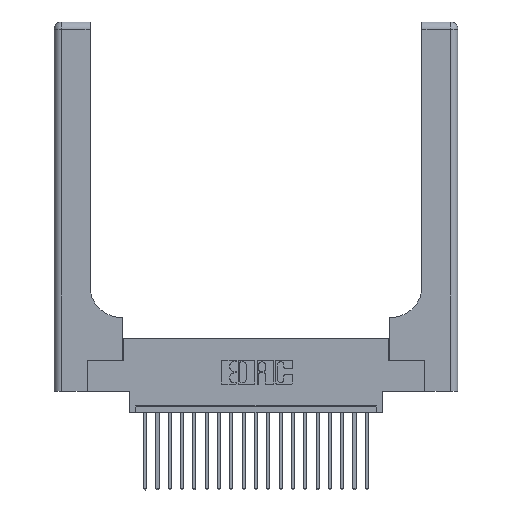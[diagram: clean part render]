
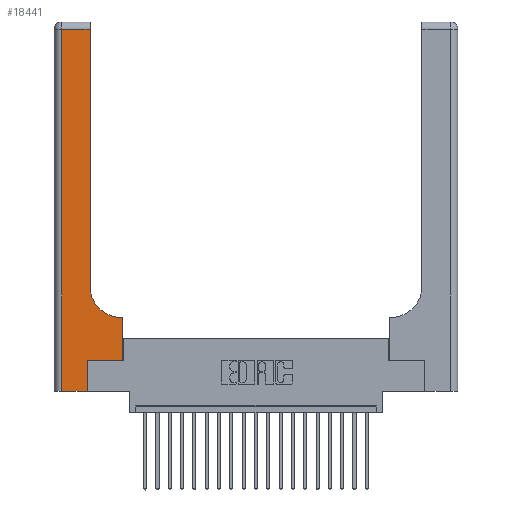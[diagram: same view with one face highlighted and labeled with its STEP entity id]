
A CAD part, top view. The second image highlights one B-rep face of the part: STEP entity #18441.
In plain terms, the highlighted planar face has unit normal (0, 0, 1).
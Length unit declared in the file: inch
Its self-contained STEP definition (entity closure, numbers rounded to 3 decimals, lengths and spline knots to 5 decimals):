
#41 = CARTESIAN_POINT ( 'NONE',  ( 0.5585, 0.25, 0.37 ) ) ;
#210 = EDGE_CURVE ( 'NONE', #21299, #14272, #16969, .T. ) ;
#269 = ORIENTED_EDGE ( 'NONE', *, *, #1497, .T. ) ;
#330 = CIRCLE ( 'NONE', #10461, 0.25 ) ;
#698 = DIRECTION ( 'NONE',  ( -1., 0., 0. ) ) ;
#745 = DIRECTION ( 'NONE',  ( 0., 0., -1. ) ) ;
#849 = CARTESIAN_POINT ( 'NONE',  ( 0.2915, 0.6, 0.37 ) ) ;
#1424 = EDGE_CURVE ( 'NONE', #20159, #21299, #2912, .T. ) ;
#1452 = DIRECTION ( 'NONE',  ( 0., 1., 0. ) ) ;
#1497 = EDGE_CURVE ( 'NONE', #2057, #20159, #17442, .T. ) ;
#2057 = VERTEX_POINT ( 'NONE', #9006 ) ;
#2519 = DIRECTION ( 'NONE',  ( 1., 0., 0. ) ) ;
#2525 = LINE ( 'NONE', #849, #6608 ) ;
#2905 = EDGE_CURVE ( 'NONE', #6541, #14317, #20978, .T. ) ;
#2912 = LINE ( 'NONE', #14805, #12250 ) ;
#2930 = EDGE_CURVE ( 'NONE', #19943, #2057, #22365, .T. ) ;
#3531 = ORIENTED_EDGE ( 'NONE', *, *, #210, .T. ) ;
#3697 = PLANE ( 'NONE',  #21068 ) ;
#4563 = VECTOR ( 'NONE', #19648, 39.37008 ) ;
#4800 = EDGE_CURVE ( 'NONE', #21307, #19943, #330, .T. ) ;
#5366 = CARTESIAN_POINT ( 'NONE',  ( 0., 3., 0.37 ) ) ;
#6043 = EDGE_LOOP ( 'NONE', ( #14001, #269, #18951, #3531, #19876, #7457, #15281, #12295, #6261 ) ) ;
#6261 = ORIENTED_EDGE ( 'NONE', *, *, #4800, .T. ) ;
#6470 = FACE_OUTER_BOUND ( 'NONE', #6043, .T. ) ;
#6541 = VERTEX_POINT ( 'NONE', #41 ) ;
#6608 = VECTOR ( 'NONE', #698, 39.37008 ) ;
#7457 = ORIENTED_EDGE ( 'NONE', *, *, #15434, .T. ) ;
#7998 = CARTESIAN_POINT ( 'NONE',  ( 0.06, 2.94, 0.37 ) ) ;
#9006 = CARTESIAN_POINT ( 'NONE',  ( 0.2915, 2.94, 0.37 ) ) ;
#10131 = CARTESIAN_POINT ( 'NONE',  ( 0.5415, 0.6, 0.37 ) ) ;
#10461 = AXIS2_PLACEMENT_3D ( 'NONE', #19965, #745, #2519 ) ;
#10603 = DIRECTION ( 'NONE',  ( 0., 1., 0. ) ) ;
#10661 = VECTOR ( 'NONE', #1452, 39.37008 ) ;
#10662 = DIRECTION ( 'NONE',  ( -1., 0., 0. ) ) ;
#11238 = CARTESIAN_POINT ( 'NONE',  ( 0.2915, 0.85, 0.37 ) ) ;
#11254 = DIRECTION ( 'NONE',  ( 0., -1., 0. ) ) ;
#11331 = LINE ( 'NONE', #11946, #16541 ) ;
#11946 = CARTESIAN_POINT ( 'NONE',  ( 0.269, 0.25, 0.37 ) ) ;
#11962 = EDGE_CURVE ( 'NONE', #14272, #17494, #19972, .T. ) ;
#12250 = VECTOR ( 'NONE', #11254, 39.37008 ) ;
#12295 = ORIENTED_EDGE ( 'NONE', *, *, #16539, .T. ) ;
#12315 = VECTOR ( 'NONE', #16467, 39.37008 ) ;
#12497 = VECTOR ( 'NONE', #10603, 39.37008 ) ;
#13168 = CARTESIAN_POINT ( 'NONE',  ( 0.5585, 0.6, 0.37 ) ) ;
#13658 = CARTESIAN_POINT ( 'NONE',  ( 0.269, 0., 0.37 ) ) ;
#14001 = ORIENTED_EDGE ( 'NONE', *, *, #2930, .T. ) ;
#14272 = VERTEX_POINT ( 'NONE', #18033 ) ;
#14317 = VERTEX_POINT ( 'NONE', #13168 ) ;
#14805 = CARTESIAN_POINT ( 'NONE',  ( 0.06, 3., 0.37 ) ) ;
#15281 = ORIENTED_EDGE ( 'NONE', *, *, #2905, .T. ) ;
#15434 = EDGE_CURVE ( 'NONE', #17494, #6541, #11331, .T. ) ;
#15770 = CARTESIAN_POINT ( 'NONE',  ( 0.2915, 3., 0.37 ) ) ;
#16467 = DIRECTION ( 'NONE',  ( 1., 0., 0. ) ) ;
#16539 = EDGE_CURVE ( 'NONE', #14317, #21307, #2525, .T. ) ;
#16541 = VECTOR ( 'NONE', #20564, 39.37008 ) ;
#16969 = LINE ( 'NONE', #21659, #12315 ) ;
#17228 = CARTESIAN_POINT ( 'NONE',  ( 0.269, 0.25, 0.37 ) ) ;
#17442 = LINE ( 'NONE', #18275, #4563 ) ;
#17494 = VERTEX_POINT ( 'NONE', #17228 ) ;
#17497 = DIRECTION ( 'NONE',  ( 0., 1., 0. ) ) ;
#17679 = VECTOR ( 'NONE', #17497, 39.37008 ) ;
#18033 = CARTESIAN_POINT ( 'NONE',  ( 0.269, 0., 0.37 ) ) ;
#18275 = CARTESIAN_POINT ( 'NONE',  ( 0., 2.94, 0.37 ) ) ;
#18441 = ADVANCED_FACE ( 'NONE', ( #6470 ), #3697, .F. ) ;
#18951 = ORIENTED_EDGE ( 'NONE', *, *, #1424, .T. ) ;
#19013 = CARTESIAN_POINT ( 'NONE',  ( 0.5585, 0.25, 0.37 ) ) ;
#19537 = DIRECTION ( 'NONE',  ( 0., 0., -1. ) ) ;
#19648 = DIRECTION ( 'NONE',  ( -1., 0., 0. ) ) ;
#19876 = ORIENTED_EDGE ( 'NONE', *, *, #11962, .T. ) ;
#19943 = VERTEX_POINT ( 'NONE', #11238 ) ;
#19965 = CARTESIAN_POINT ( 'NONE',  ( 0.5415, 0.85, 0.37 ) ) ;
#19972 = LINE ( 'NONE', #13658, #10661 ) ;
#20159 = VERTEX_POINT ( 'NONE', #7998 ) ;
#20564 = DIRECTION ( 'NONE',  ( 1., 0., 0. ) ) ;
#20760 = CARTESIAN_POINT ( 'NONE',  ( 0.06, 0., 0.37 ) ) ;
#20978 = LINE ( 'NONE', #19013, #12497 ) ;
#21068 = AXIS2_PLACEMENT_3D ( 'NONE', #5366, #19537, #10662 ) ;
#21299 = VERTEX_POINT ( 'NONE', #20760 ) ;
#21307 = VERTEX_POINT ( 'NONE', #10131 ) ;
#21659 = CARTESIAN_POINT ( 'NONE',  ( 0., 0., 0.37 ) ) ;
#22365 = LINE ( 'NONE', #15770, #17679 ) ;
